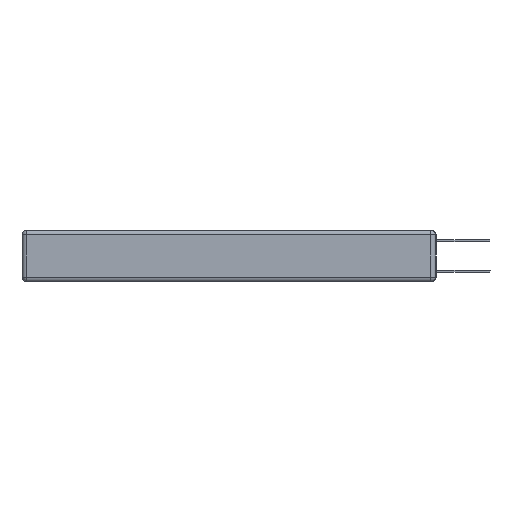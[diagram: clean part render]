
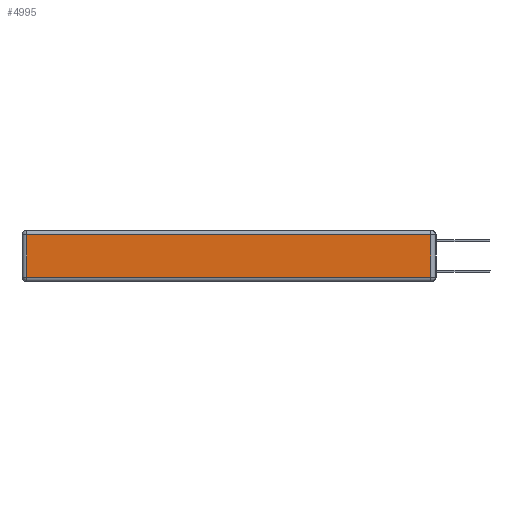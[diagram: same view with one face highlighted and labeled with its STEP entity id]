
A CAD part, left-side view. The second image highlights one B-rep face of the part: STEP entity #4995.
In plain terms, the highlighted planar face has unit normal (-1, 0, 0).
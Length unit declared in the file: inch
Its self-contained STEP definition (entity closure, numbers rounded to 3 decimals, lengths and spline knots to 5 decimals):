
#295 = ORIENTED_EDGE ( 'NONE', *, *, #9350, .T. ) ;
#488 = DIRECTION ( 'NONE',  ( 0., 0., 1. ) ) ;
#873 = DIRECTION ( 'NONE',  ( 0., 1., 0. ) ) ;
#1420 = VECTOR ( 'NONE', #488, 39.37008 ) ;
#1814 = LINE ( 'NONE', #3395, #2222 ) ;
#1887 = PLANE ( 'NONE',  #4610 ) ;
#2222 = VECTOR ( 'NONE', #873, 39.37008 ) ;
#2749 = FACE_OUTER_BOUND ( 'NONE', #3571, .T. ) ;
#3395 = CARTESIAN_POINT ( 'NONE',  ( 0., 2.75, -0.03 ) ) ;
#3571 = EDGE_LOOP ( 'NONE', ( #7034, #14503, #295, #8843 ) ) ;
#4277 = DIRECTION ( 'NONE',  ( 0., 0., -1. ) ) ;
#4366 = CARTESIAN_POINT ( 'NONE',  ( 0., 0., -0.313 ) ) ;
#4610 = AXIS2_PLACEMENT_3D ( 'NONE', #5673, #11283, #15284 ) ;
#4995 = ADVANCED_FACE ( 'NONE', ( #2749 ), #1887, .T. ) ;
#5429 = EDGE_CURVE ( 'NONE', #8371, #9354, #6036, .T. ) ;
#5673 = CARTESIAN_POINT ( 'NONE',  ( 0., 0., -0.343 ) ) ;
#6036 = LINE ( 'NONE', #4366, #14756 ) ;
#6750 = LINE ( 'NONE', #8320, #1420 ) ;
#6987 = CARTESIAN_POINT ( 'NONE',  ( 0., 0.03, -0.03 ) ) ;
#7034 = ORIENTED_EDGE ( 'NONE', *, *, #5429, .T. ) ;
#8249 = CARTESIAN_POINT ( 'NONE',  ( 0., 2.72, -0.343 ) ) ;
#8320 = CARTESIAN_POINT ( 'NONE',  ( 0., 0.03, -0.343 ) ) ;
#8343 = DIRECTION ( 'NONE',  ( 0., -1., 0. ) ) ;
#8371 = VERTEX_POINT ( 'NONE', #12131 ) ;
#8843 = ORIENTED_EDGE ( 'NONE', *, *, #9083, .T. ) ;
#9083 = EDGE_CURVE ( 'NONE', #13722, #8371, #12340, .T. ) ;
#9350 = EDGE_CURVE ( 'NONE', #11910, #13722, #1814, .T. ) ;
#9354 = VERTEX_POINT ( 'NONE', #14155 ) ;
#11283 = DIRECTION ( 'NONE',  ( -1., 0., 0. ) ) ;
#11740 = CARTESIAN_POINT ( 'NONE',  ( 0., 2.72, -0.03 ) ) ;
#11910 = VERTEX_POINT ( 'NONE', #6987 ) ;
#12110 = VECTOR ( 'NONE', #4277, 39.37008 ) ;
#12131 = CARTESIAN_POINT ( 'NONE',  ( 0., 2.72, -0.313 ) ) ;
#12340 = LINE ( 'NONE', #8249, #12110 ) ;
#13722 = VERTEX_POINT ( 'NONE', #11740 ) ;
#14155 = CARTESIAN_POINT ( 'NONE',  ( 0., 0.03, -0.313 ) ) ;
#14503 = ORIENTED_EDGE ( 'NONE', *, *, #16150, .T. ) ;
#14756 = VECTOR ( 'NONE', #8343, 39.37008 ) ;
#15284 = DIRECTION ( 'NONE',  ( 0., 0., 1. ) ) ;
#16150 = EDGE_CURVE ( 'NONE', #9354, #11910, #6750, .T. ) ;
